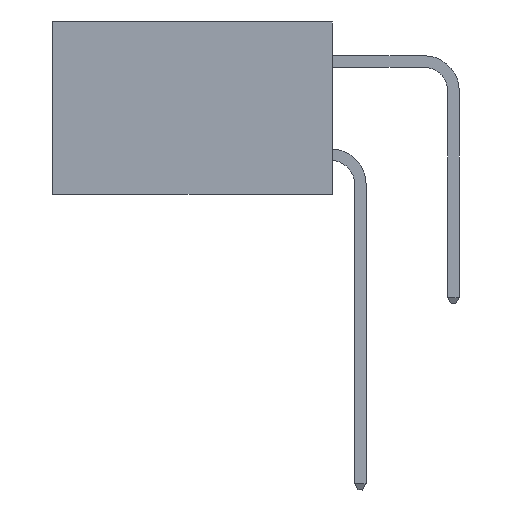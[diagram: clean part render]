
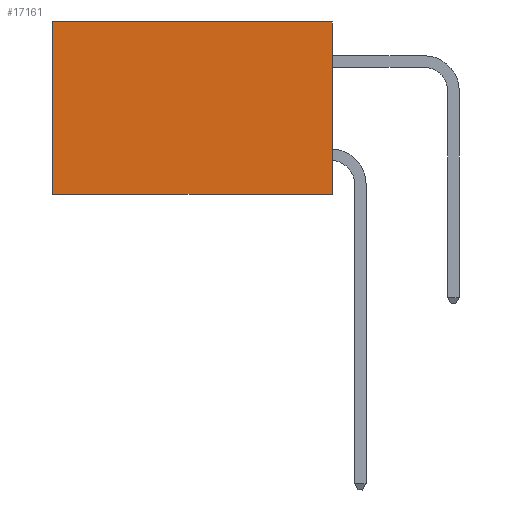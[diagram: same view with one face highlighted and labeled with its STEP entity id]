
A CAD part, left-side view. The second image highlights one B-rep face of the part: STEP entity #17161.
In plain terms, the highlighted planar face has unit normal (-1, 0, 0).
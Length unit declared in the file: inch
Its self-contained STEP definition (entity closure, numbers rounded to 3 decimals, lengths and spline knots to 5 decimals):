
#380 = VECTOR ( 'NONE', #15399, 39.37008 ) ;
#626 = ORIENTED_EDGE ( 'NONE', *, *, #1665, .T. ) ;
#1665 = EDGE_CURVE ( 'NONE', #10802, #23105, #4589, .T. ) ;
#3033 = VECTOR ( 'NONE', #22860, 39.37008 ) ;
#3161 = EDGE_CURVE ( 'NONE', #5676, #10881, #13947, .T. ) ;
#4473 = CARTESIAN_POINT ( 'NONE',  ( 0.2615, 0., 0. ) ) ;
#4589 = LINE ( 'NONE', #4473, #21260 ) ;
#4807 = DIRECTION ( 'NONE',  ( 0., 0., -1. ) ) ;
#5676 = VERTEX_POINT ( 'NONE', #12544 ) ;
#6883 = EDGE_CURVE ( 'NONE', #10802, #5676, #22648, .T. ) ;
#7811 = CARTESIAN_POINT ( 'NONE',  ( 0.2615, 0., -0.37 ) ) ;
#9963 = CARTESIAN_POINT ( 'NONE',  ( 0.2615, 0., -0.37 ) ) ;
#10197 = CARTESIAN_POINT ( 'NONE',  ( 0.2615, 0.6, 0. ) ) ;
#10246 = FACE_OUTER_BOUND ( 'NONE', #11981, .T. ) ;
#10713 = AXIS2_PLACEMENT_3D ( 'NONE', #7811, #15032, #22272 ) ;
#10802 = VERTEX_POINT ( 'NONE', #19461 ) ;
#10881 = VERTEX_POINT ( 'NONE', #14359 ) ;
#11981 = EDGE_LOOP ( 'NONE', ( #21610, #12858, #15855, #626 ) ) ;
#12544 = CARTESIAN_POINT ( 'NONE',  ( 0.2615, 0., -0.37 ) ) ;
#12568 = VECTOR ( 'NONE', #4807, 39.37008 ) ;
#12858 = ORIENTED_EDGE ( 'NONE', *, *, #3161, .F. ) ;
#13798 = LINE ( 'NONE', #21030, #12568 ) ;
#13947 = LINE ( 'NONE', #19766, #3033 ) ;
#14359 = CARTESIAN_POINT ( 'NONE',  ( 0.2615, 0.6, -0.37 ) ) ;
#15032 = DIRECTION ( 'NONE',  ( 1., 0., 0. ) ) ;
#15399 = DIRECTION ( 'NONE',  ( 0., 0., -1. ) ) ;
#15833 = EDGE_CURVE ( 'NONE', #23105, #10881, #13798, .T. ) ;
#15855 = ORIENTED_EDGE ( 'NONE', *, *, #6883, .F. ) ;
#17161 = ADVANCED_FACE ( 'NONE', ( #10246 ), #17487, .F. ) ;
#17487 = PLANE ( 'NONE',  #10713 ) ;
#19461 = CARTESIAN_POINT ( 'NONE',  ( 0.2615, 0., 0. ) ) ;
#19766 = CARTESIAN_POINT ( 'NONE',  ( 0.2615, 0., -0.37 ) ) ;
#21030 = CARTESIAN_POINT ( 'NONE',  ( 0.2615, 0.6, -0.37 ) ) ;
#21260 = VECTOR ( 'NONE', #22709, 39.37008 ) ;
#21610 = ORIENTED_EDGE ( 'NONE', *, *, #15833, .T. ) ;
#22272 = DIRECTION ( 'NONE',  ( 0., 0., -1. ) ) ;
#22648 = LINE ( 'NONE', #9963, #380 ) ;
#22709 = DIRECTION ( 'NONE',  ( 0., 1., 0. ) ) ;
#22860 = DIRECTION ( 'NONE',  ( 0., 1., 0. ) ) ;
#23105 = VERTEX_POINT ( 'NONE', #10197 ) ;
